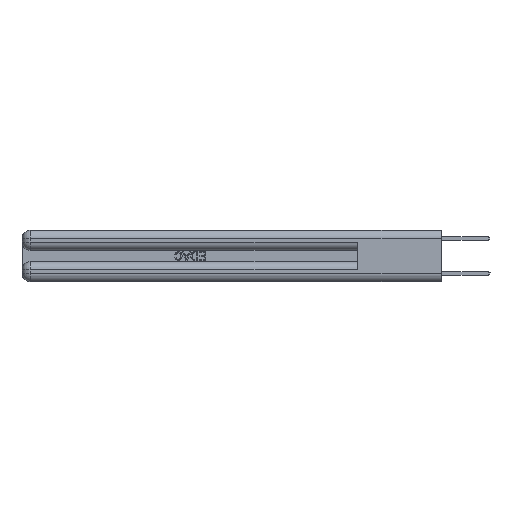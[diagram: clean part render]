
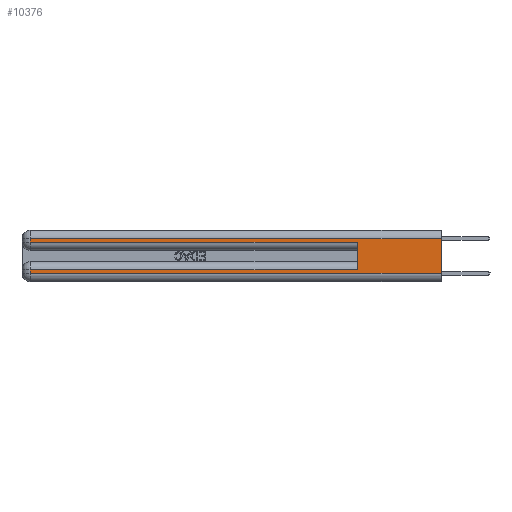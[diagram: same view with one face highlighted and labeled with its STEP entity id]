
A CAD part, left-side view. The second image highlights one B-rep face of the part: STEP entity #10376.
In plain terms, the highlighted planar face has unit normal (-1, 0, 0).
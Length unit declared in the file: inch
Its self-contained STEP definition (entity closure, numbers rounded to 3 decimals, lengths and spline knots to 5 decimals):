
#173 = CARTESIAN_POINT ( 'NONE',  ( 0., 0., 0.06 ) ) ;
#901 = LINE ( 'NONE', #27133, #20480 ) ;
#939 = DIRECTION ( 'NONE',  ( 0., 0., -1. ) ) ;
#1540 = DIRECTION ( 'NONE',  ( 0., 0., -1. ) ) ;
#1566 = EDGE_CURVE ( 'NONE', #26423, #15707, #20767, .T. ) ;
#1771 = LINE ( 'NONE', #18493, #2445 ) ;
#2258 = EDGE_CURVE ( 'NONE', #12378, #19068, #19381, .T. ) ;
#2445 = VECTOR ( 'NONE', #7808, 39.37008 ) ;
#2469 = LINE ( 'NONE', #4348, #24761 ) ;
#2655 = CARTESIAN_POINT ( 'NONE',  ( 0., 0., 0.37 ) ) ;
#2727 = DIRECTION ( 'NONE',  ( 0., -1., 0. ) ) ;
#4185 = CARTESIAN_POINT ( 'NONE',  ( 0., 2.94, 0.06 ) ) ;
#4219 = ORIENTED_EDGE ( 'NONE', *, *, #8422, .T. ) ;
#4348 = CARTESIAN_POINT ( 'NONE',  ( 0., 0., 0.085 ) ) ;
#4822 = DIRECTION ( 'NONE',  ( 0., 0., -1. ) ) ;
#4968 = VERTEX_POINT ( 'NONE', #15204 ) ;
#7002 = CARTESIAN_POINT ( 'NONE',  ( 0., 2.94, 0.285 ) ) ;
#7808 = DIRECTION ( 'NONE',  ( 0., 1., 0. ) ) ;
#8422 = EDGE_CURVE ( 'NONE', #11779, #23478, #2469, .T. ) ;
#9418 = LINE ( 'NONE', #22644, #20173 ) ;
#10376 = ADVANCED_FACE ( 'NONE', ( #11500 ), #24059, .F. ) ;
#11053 = ORIENTED_EDGE ( 'NONE', *, *, #2258, .T. ) ;
#11136 = CARTESIAN_POINT ( 'NONE',  ( 0., 0., 0.06 ) ) ;
#11143 = DIRECTION ( 'NONE',  ( 1., 0., 0. ) ) ;
#11331 = VECTOR ( 'NONE', #1540, 39.37008 ) ;
#11500 = FACE_OUTER_BOUND ( 'NONE', #16955, .T. ) ;
#11737 = VECTOR ( 'NONE', #16027, 39.37008 ) ;
#11779 = VERTEX_POINT ( 'NONE', #18390 ) ;
#11824 = DIRECTION ( 'NONE',  ( 0., 0., 1. ) ) ;
#12068 = EDGE_CURVE ( 'NONE', #15707, #4968, #21154, .T. ) ;
#12141 = DIRECTION ( 'NONE',  ( 0., 0., -1. ) ) ;
#12184 = EDGE_CURVE ( 'NONE', #19926, #19068, #13129, .T. ) ;
#12378 = VERTEX_POINT ( 'NONE', #4185 ) ;
#12733 = EDGE_CURVE ( 'NONE', #11779, #4968, #9418, .T. ) ;
#13129 = LINE ( 'NONE', #2655, #16151 ) ;
#13318 = EDGE_CURVE ( 'NONE', #23478, #12378, #901, .T. ) ;
#14356 = VECTOR ( 'NONE', #2727, 39.37008 ) ;
#15204 = CARTESIAN_POINT ( 'NONE',  ( 0., 0.6, 0.285 ) ) ;
#15511 = CARTESIAN_POINT ( 'NONE',  ( 0., 0., 0.37 ) ) ;
#15707 = VERTEX_POINT ( 'NONE', #7002 ) ;
#15842 = AXIS2_PLACEMENT_3D ( 'NONE', #15511, #11143, #4822 ) ;
#16027 = DIRECTION ( 'NONE',  ( 0., -1., 0. ) ) ;
#16151 = VECTOR ( 'NONE', #939, 39.37008 ) ;
#16955 = EDGE_LOOP ( 'NONE', ( #20444, #18351, #23121, #26667, #24750, #4219, #25763, #11053 ) ) ;
#18351 = ORIENTED_EDGE ( 'NONE', *, *, #20659, .T. ) ;
#18390 = CARTESIAN_POINT ( 'NONE',  ( 0., 0.6, 0.085 ) ) ;
#18493 = CARTESIAN_POINT ( 'NONE',  ( 0., 0., 0.31 ) ) ;
#19068 = VERTEX_POINT ( 'NONE', #173 ) ;
#19381 = LINE ( 'NONE', #11136, #14356 ) ;
#19781 = CARTESIAN_POINT ( 'NONE',  ( 0., 2.94, 0.37 ) ) ;
#19926 = VERTEX_POINT ( 'NONE', #22169 ) ;
#20173 = VECTOR ( 'NONE', #11824, 39.37008 ) ;
#20444 = ORIENTED_EDGE ( 'NONE', *, *, #12184, .F. ) ;
#20480 = VECTOR ( 'NONE', #12141, 39.37008 ) ;
#20659 = EDGE_CURVE ( 'NONE', #19926, #26423, #1771, .T. ) ;
#20767 = LINE ( 'NONE', #19781, #11331 ) ;
#21154 = LINE ( 'NONE', #26926, #11737 ) ;
#22169 = CARTESIAN_POINT ( 'NONE',  ( 0., 0., 0.31 ) ) ;
#22644 = CARTESIAN_POINT ( 'NONE',  ( 0., 0.6, 0.145 ) ) ;
#23121 = ORIENTED_EDGE ( 'NONE', *, *, #1566, .T. ) ;
#23478 = VERTEX_POINT ( 'NONE', #27531 ) ;
#23520 = CARTESIAN_POINT ( 'NONE',  ( 0., 2.94, 0.31 ) ) ;
#24059 = PLANE ( 'NONE',  #15842 ) ;
#24750 = ORIENTED_EDGE ( 'NONE', *, *, #12733, .F. ) ;
#24761 = VECTOR ( 'NONE', #27933, 39.37008 ) ;
#25763 = ORIENTED_EDGE ( 'NONE', *, *, #13318, .T. ) ;
#26423 = VERTEX_POINT ( 'NONE', #23520 ) ;
#26667 = ORIENTED_EDGE ( 'NONE', *, *, #12068, .T. ) ;
#26926 = CARTESIAN_POINT ( 'NONE',  ( 0., 0., 0.285 ) ) ;
#27133 = CARTESIAN_POINT ( 'NONE',  ( 0., 2.94, 0.37 ) ) ;
#27531 = CARTESIAN_POINT ( 'NONE',  ( 0., 2.94, 0.085 ) ) ;
#27933 = DIRECTION ( 'NONE',  ( 0., 1., 0. ) ) ;
